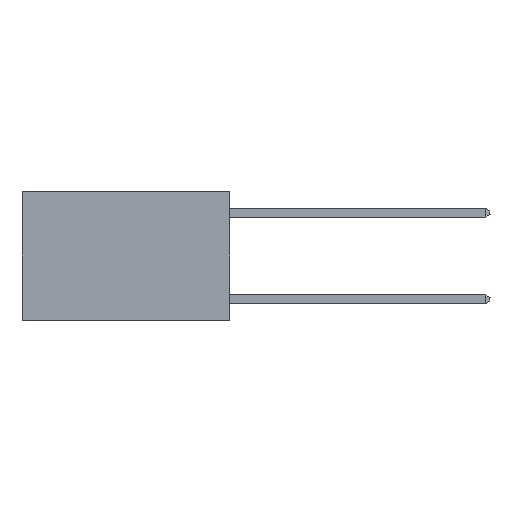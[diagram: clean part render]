
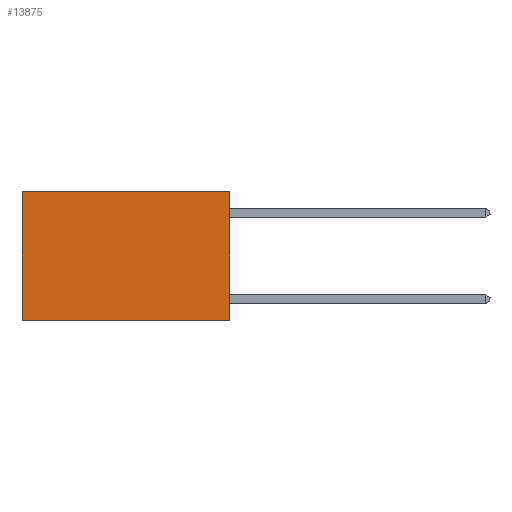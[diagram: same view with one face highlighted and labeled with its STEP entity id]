
A CAD part, left-side view. The second image highlights one B-rep face of the part: STEP entity #13875.
In plain terms, the highlighted planar face has unit normal (-1, 0, 0).
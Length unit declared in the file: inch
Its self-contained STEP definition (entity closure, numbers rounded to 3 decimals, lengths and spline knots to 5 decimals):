
#265 = CARTESIAN_POINT ( 'NONE',  ( 0.2625, 0., -0.37 ) ) ;
#504 = LINE ( 'NONE', #265, #23914 ) ;
#1672 = EDGE_CURVE ( 'NONE', #5755, #6637, #8775, .T. ) ;
#2754 = VECTOR ( 'NONE', #13678, 39.37008 ) ;
#2756 = CARTESIAN_POINT ( 'NONE',  ( 0.2625, 0.6, 0. ) ) ;
#2768 = ORIENTED_EDGE ( 'NONE', *, *, #6463, .F. ) ;
#2776 = DIRECTION ( 'NONE',  ( 0., 0., -1. ) ) ;
#4021 = CARTESIAN_POINT ( 'NONE',  ( 0.2625, 0., 0. ) ) ;
#4072 = EDGE_LOOP ( 'NONE', ( #15393, #9784, #2768, #20557 ) ) ;
#5072 = CARTESIAN_POINT ( 'NONE',  ( 0.2625, 0., 0. ) ) ;
#5602 = PLANE ( 'NONE',  #10316 ) ;
#5755 = VERTEX_POINT ( 'NONE', #2756 ) ;
#5774 = VERTEX_POINT ( 'NONE', #16709 ) ;
#6263 = VECTOR ( 'NONE', #2776, 39.37008 ) ;
#6463 = EDGE_CURVE ( 'NONE', #5774, #21950, #19078, .T. ) ;
#6637 = VERTEX_POINT ( 'NONE', #12023 ) ;
#7058 = EDGE_CURVE ( 'NONE', #21950, #6637, #504, .T. ) ;
#8040 = DIRECTION ( 'NONE',  ( 0., 1., 0. ) ) ;
#8775 = LINE ( 'NONE', #23865, #6263 ) ;
#8926 = VECTOR ( 'NONE', #9284, 39.37008 ) ;
#9284 = DIRECTION ( 'NONE',  ( 0., 0., -1. ) ) ;
#9784 = ORIENTED_EDGE ( 'NONE', *, *, #7058, .F. ) ;
#10316 = AXIS2_PLACEMENT_3D ( 'NONE', #5072, #12974, #20968 ) ;
#12023 = CARTESIAN_POINT ( 'NONE',  ( 0.2625, 0.6, -0.37 ) ) ;
#12974 = DIRECTION ( 'NONE',  ( 1., 0., 0. ) ) ;
#13678 = DIRECTION ( 'NONE',  ( 0., 1., 0. ) ) ;
#13875 = ADVANCED_FACE ( 'NONE', ( #15406 ), #5602, .F. ) ;
#15393 = ORIENTED_EDGE ( 'NONE', *, *, #1672, .T. ) ;
#15406 = FACE_OUTER_BOUND ( 'NONE', #4072, .T. ) ;
#15847 = LINE ( 'NONE', #4021, #2754 ) ;
#16709 = CARTESIAN_POINT ( 'NONE',  ( 0.2625, 0., 0. ) ) ;
#16852 = CARTESIAN_POINT ( 'NONE',  ( 0.2625, 0., -0.37 ) ) ;
#19078 = LINE ( 'NONE', #19203, #8926 ) ;
#19203 = CARTESIAN_POINT ( 'NONE',  ( 0.2625, 0., 0. ) ) ;
#20557 = ORIENTED_EDGE ( 'NONE', *, *, #25017, .T. ) ;
#20968 = DIRECTION ( 'NONE',  ( 0., 0., -1. ) ) ;
#21950 = VERTEX_POINT ( 'NONE', #16852 ) ;
#23865 = CARTESIAN_POINT ( 'NONE',  ( 0.2625, 0.6, 0. ) ) ;
#23914 = VECTOR ( 'NONE', #8040, 39.37008 ) ;
#25017 = EDGE_CURVE ( 'NONE', #5774, #5755, #15847, .T. ) ;
